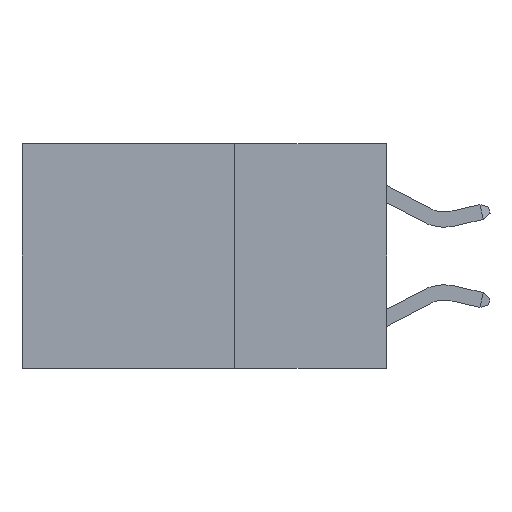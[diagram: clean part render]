
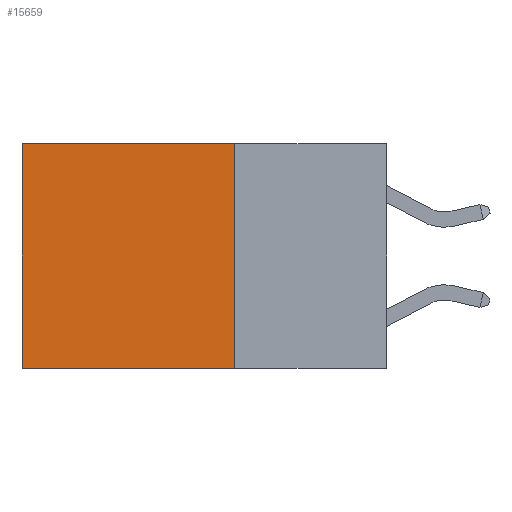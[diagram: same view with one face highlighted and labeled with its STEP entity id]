
A CAD part, left-side view. The second image highlights one B-rep face of the part: STEP entity #15659.
In plain terms, the highlighted planar face has unit normal (-1, 0, 0).
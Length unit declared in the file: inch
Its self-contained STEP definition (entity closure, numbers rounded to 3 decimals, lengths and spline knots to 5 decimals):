
#98 = EDGE_CURVE ( 'NONE', #23678, #11198, #8414, .T. ) ;
#2528 = LINE ( 'NONE', #19597, #4288 ) ;
#3153 = VECTOR ( 'NONE', #6394, 39.37008 ) ;
#4288 = VECTOR ( 'NONE', #17829, 39.37008 ) ;
#4498 = CARTESIAN_POINT ( 'NONE',  ( 0.2625, 0.25, 0. ) ) ;
#5224 = EDGE_CURVE ( 'NONE', #23678, #5587, #21201, .T. ) ;
#5587 = VERTEX_POINT ( 'NONE', #15273 ) ;
#6394 = DIRECTION ( 'NONE',  ( 0., 1., 0. ) ) ;
#6671 = CARTESIAN_POINT ( 'NONE',  ( 0.2625, 0.6, 0. ) ) ;
#6911 = VECTOR ( 'NONE', #11799, 39.37008 ) ;
#8414 = LINE ( 'NONE', #4498, #3153 ) ;
#9670 = PLANE ( 'NONE',  #10470 ) ;
#10156 = CARTESIAN_POINT ( 'NONE',  ( 0.2625, 0.25, 0. ) ) ;
#10470 = AXIS2_PLACEMENT_3D ( 'NONE', #17510, #21460, #13452 ) ;
#10591 = EDGE_CURVE ( 'NONE', #5587, #23228, #2528, .T. ) ;
#11198 = VERTEX_POINT ( 'NONE', #6671 ) ;
#11558 = FACE_OUTER_BOUND ( 'NONE', #23346, .T. ) ;
#11799 = DIRECTION ( 'NONE',  ( 0., 0., -1. ) ) ;
#13452 = DIRECTION ( 'NONE',  ( 0., 0., -1. ) ) ;
#14954 = ORIENTED_EDGE ( 'NONE', *, *, #5224, .F. ) ;
#15273 = CARTESIAN_POINT ( 'NONE',  ( 0.2625, 0.25, -0.37 ) ) ;
#15429 = CARTESIAN_POINT ( 'NONE',  ( 0.2625, 0.25, 0. ) ) ;
#15659 = ADVANCED_FACE ( 'NONE', ( #11558 ), #9670, .F. ) ;
#16205 = VECTOR ( 'NONE', #22556, 39.37008 ) ;
#16731 = CARTESIAN_POINT ( 'NONE',  ( 0.2625, 0.6, 0. ) ) ;
#17510 = CARTESIAN_POINT ( 'NONE',  ( 0.2625, 0.25, 0. ) ) ;
#17829 = DIRECTION ( 'NONE',  ( 0., 1., 0. ) ) ;
#19597 = CARTESIAN_POINT ( 'NONE',  ( 0.2625, 0.25, -0.37 ) ) ;
#20926 = ORIENTED_EDGE ( 'NONE', *, *, #98, .T. ) ;
#21076 = CARTESIAN_POINT ( 'NONE',  ( 0.2625, 0.6, -0.37 ) ) ;
#21201 = LINE ( 'NONE', #10156, #6911 ) ;
#21460 = DIRECTION ( 'NONE',  ( 1., 0., 0. ) ) ;
#22556 = DIRECTION ( 'NONE',  ( 0., 0., -1. ) ) ;
#23228 = VERTEX_POINT ( 'NONE', #21076 ) ;
#23346 = EDGE_LOOP ( 'NONE', ( #24760, #24024, #14954, #20926 ) ) ;
#23678 = VERTEX_POINT ( 'NONE', #15429 ) ;
#24024 = ORIENTED_EDGE ( 'NONE', *, *, #10591, .F. ) ;
#24318 = LINE ( 'NONE', #16731, #16205 ) ;
#24760 = ORIENTED_EDGE ( 'NONE', *, *, #24915, .T. ) ;
#24915 = EDGE_CURVE ( 'NONE', #11198, #23228, #24318, .T. ) ;
